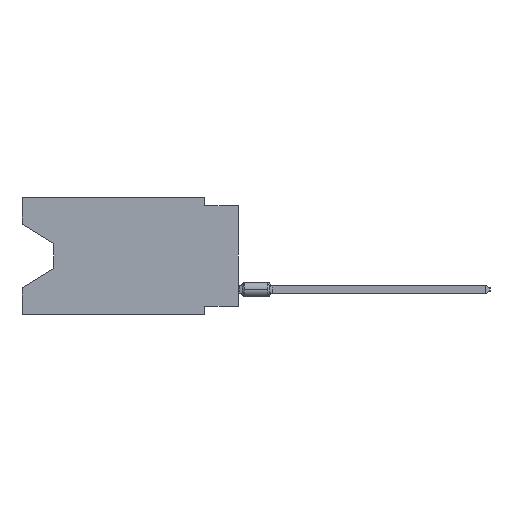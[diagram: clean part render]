
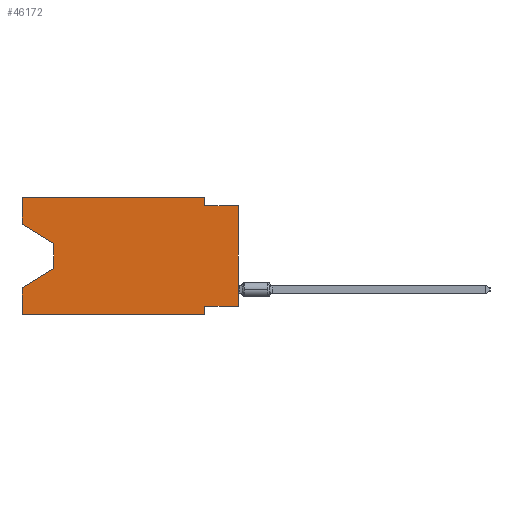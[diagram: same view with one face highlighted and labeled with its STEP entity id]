
A CAD part, left-side view. The second image highlights one B-rep face of the part: STEP entity #46172.
In plain terms, the highlighted planar face has unit normal (-1, 0, 0).
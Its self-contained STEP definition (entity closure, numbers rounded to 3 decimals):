
#573 = CARTESIAN_POINT ( 'NONE',  ( 0., 16.383, 0. ) ) ;
#797 = CARTESIAN_POINT ( 'NONE',  ( 0., 0., 0. ) ) ;
#1622 = FACE_OUTER_BOUND ( 'NONE', #34906, .T. ) ;
#1699 = ORIENTED_EDGE ( 'NONE', *, *, #53147, .F. ) ;
#1901 = ORIENTED_EDGE ( 'NONE', *, *, #46007, .F. ) ;
#3218 = VECTOR ( 'NONE', #59143, 1000. ) ;
#4753 = CARTESIAN_POINT ( 'NONE',  ( 0., 2.54, -8.89 ) ) ;
#4857 = ORIENTED_EDGE ( 'NONE', *, *, #44909, .F. ) ;
#4880 = CARTESIAN_POINT ( 'NONE',  ( 0., 2.54, -8.255 ) ) ;
#5239 = VERTEX_POINT ( 'NONE', #45162 ) ;
#5913 = DIRECTION ( 'NONE',  ( 0., 0., -1. ) ) ;
#6599 = VECTOR ( 'NONE', #42693, 1000. ) ;
#9286 = VERTEX_POINT ( 'NONE', #69932 ) ;
#9695 = LINE ( 'NONE', #57560, #27453 ) ;
#13387 = LINE ( 'NONE', #573, #32443 ) ;
#13675 = DIRECTION ( 'NONE',  ( 0., 0.855, -0.519 ) ) ;
#13773 = ORIENTED_EDGE ( 'NONE', *, *, #48867, .T. ) ;
#15728 = EDGE_CURVE ( 'NONE', #70137, #43646, #58070, .T. ) ;
#15932 = DIRECTION ( 'NONE',  ( 0., -1., 0. ) ) ;
#17198 = CARTESIAN_POINT ( 'NONE',  ( 0., 16.383, 0. ) ) ;
#17421 = CARTESIAN_POINT ( 'NONE',  ( 0., 16.383, 0. ) ) ;
#17862 = ORIENTED_EDGE ( 'NONE', *, *, #40400, .T. ) ;
#17984 = CARTESIAN_POINT ( 'NONE',  ( 0., 13.97, -5.385 ) ) ;
#18356 = DIRECTION ( 'NONE',  ( 0., 0., 1. ) ) ;
#19121 = CARTESIAN_POINT ( 'NONE',  ( 0., 16.383, 0. ) ) ;
#20349 = CARTESIAN_POINT ( 'NONE',  ( 0., 13.97, -3.505 ) ) ;
#23929 = VERTEX_POINT ( 'NONE', #45137 ) ;
#24538 = DIRECTION ( 'NONE',  ( 0., 0., 1. ) ) ;
#25149 = VERTEX_POINT ( 'NONE', #27249 ) ;
#26267 = VECTOR ( 'NONE', #41177, 1000. ) ;
#26538 = EDGE_CURVE ( 'NONE', #53308, #5239, #53725, .T. ) ;
#27249 = CARTESIAN_POINT ( 'NONE',  ( 0., 13.97, -5.385 ) ) ;
#27453 = VECTOR ( 'NONE', #15932, 1000. ) ;
#30924 = VECTOR ( 'NONE', #5913, 1000. ) ;
#32443 = VECTOR ( 'NONE', #37129, 1000. ) ;
#32713 = ORIENTED_EDGE ( 'NONE', *, *, #26538, .F. ) ;
#34519 = ORIENTED_EDGE ( 'NONE', *, *, #42650, .F. ) ;
#34906 = EDGE_LOOP ( 'NONE', ( #13773, #42897, #68142, #4857, #58822, #54046, #1901, #17862, #32713, #66331, #34519, #1699 ) ) ;
#37129 = DIRECTION ( 'NONE',  ( 0., -1., 0. ) ) ;
#40400 = EDGE_CURVE ( 'NONE', #71248, #5239, #59157, .T. ) ;
#40989 = VECTOR ( 'NONE', #24538, 1000. ) ;
#41177 = DIRECTION ( 'NONE',  ( 0., 0., 1. ) ) ;
#41263 = LINE ( 'NONE', #53324, #3218 ) ;
#42650 = EDGE_CURVE ( 'NONE', #49979, #69189, #13387, .T. ) ;
#42693 = DIRECTION ( 'NONE',  ( 0., 1., 0. ) ) ;
#42897 = ORIENTED_EDGE ( 'NONE', *, *, #61848, .T. ) ;
#42988 = EDGE_CURVE ( 'NONE', #25149, #9286, #54547, .T. ) ;
#43270 = DIRECTION ( 'NONE',  ( 0., 0., -1. ) ) ;
#43273 = CARTESIAN_POINT ( 'NONE',  ( 0., 2.54, -0.635 ) ) ;
#43646 = VERTEX_POINT ( 'NONE', #53907 ) ;
#44909 = EDGE_CURVE ( 'NONE', #23929, #9286, #70735, .T. ) ;
#45137 = CARTESIAN_POINT ( 'NONE',  ( 0., 16.383, -8.89 ) ) ;
#45162 = CARTESIAN_POINT ( 'NONE',  ( 0., 0., -0.635 ) ) ;
#45393 = DIRECTION ( 'NONE',  ( 0., 0., -1. ) ) ;
#46007 = EDGE_CURVE ( 'NONE', #71248, #70137, #71869, .T. ) ;
#46172 = ADVANCED_FACE ( 'NONE', ( #1622 ), #48698, .F. ) ;
#48264 = CARTESIAN_POINT ( 'NONE',  ( 0., 0., -0.635 ) ) ;
#48698 = PLANE ( 'NONE',  #62473 ) ;
#48867 = EDGE_CURVE ( 'NONE', #67295, #50625, #41263, .T. ) ;
#49087 = DIRECTION ( 'NONE',  ( 1., 0., 0. ) ) ;
#49979 = VERTEX_POINT ( 'NONE', #17198 ) ;
#50625 = VERTEX_POINT ( 'NONE', #20349 ) ;
#53147 = EDGE_CURVE ( 'NONE', #67295, #49979, #71288, .T. ) ;
#53308 = VERTEX_POINT ( 'NONE', #43273 ) ;
#53324 = CARTESIAN_POINT ( 'NONE',  ( 0., 16.383, -2.038 ) ) ;
#53725 = LINE ( 'NONE', #48264, #71675 ) ;
#53907 = CARTESIAN_POINT ( 'NONE',  ( 0., 2.54, -8.89 ) ) ;
#54046 = ORIENTED_EDGE ( 'NONE', *, *, #15728, .F. ) ;
#54547 = LINE ( 'NONE', #17984, #74517 ) ;
#55778 = VECTOR ( 'NONE', #18356, 1000. ) ;
#56855 = CARTESIAN_POINT ( 'NONE',  ( 0., 2.54, 0. ) ) ;
#57560 = CARTESIAN_POINT ( 'NONE',  ( 0., 16.383, -8.89 ) ) ;
#58070 = LINE ( 'NONE', #4753, #30924 ) ;
#58822 = ORIENTED_EDGE ( 'NONE', *, *, #74525, .T. ) ;
#58921 = CARTESIAN_POINT ( 'NONE',  ( 0., 16.383, -2.038 ) ) ;
#59143 = DIRECTION ( 'NONE',  ( 0., -0.855, -0.519 ) ) ;
#59157 = LINE ( 'NONE', #797, #40989 ) ;
#59520 = EDGE_CURVE ( 'NONE', #69189, #53308, #70966, .T. ) ;
#59994 = CARTESIAN_POINT ( 'NONE',  ( 0., 16.383, 0. ) ) ;
#61735 = VECTOR ( 'NONE', #45393, 1000. ) ;
#61848 = EDGE_CURVE ( 'NONE', #50625, #25149, #69508, .T. ) ;
#62473 = AXIS2_PLACEMENT_3D ( 'NONE', #19121, #49087, #43270 ) ;
#64355 = DIRECTION ( 'NONE',  ( 0., 0., -1. ) ) ;
#64430 = CARTESIAN_POINT ( 'NONE',  ( 0., 13.97, -3.505 ) ) ;
#65195 = VECTOR ( 'NONE', #64355, 1000. ) ;
#66331 = ORIENTED_EDGE ( 'NONE', *, *, #59520, .F. ) ;
#67295 = VERTEX_POINT ( 'NONE', #58921 ) ;
#68142 = ORIENTED_EDGE ( 'NONE', *, *, #42988, .T. ) ;
#69189 = VERTEX_POINT ( 'NONE', #56855 ) ;
#69508 = LINE ( 'NONE', #64430, #61735 ) ;
#69932 = CARTESIAN_POINT ( 'NONE',  ( 0., 16.383, -6.852 ) ) ;
#69965 = CARTESIAN_POINT ( 'NONE',  ( 0., 0., -8.255 ) ) ;
#70137 = VERTEX_POINT ( 'NONE', #4880 ) ;
#70735 = LINE ( 'NONE', #17421, #26267 ) ;
#70966 = LINE ( 'NONE', #76027, #65195 ) ;
#71248 = VERTEX_POINT ( 'NONE', #69965 ) ;
#71288 = LINE ( 'NONE', #59994, #55778 ) ;
#71675 = VECTOR ( 'NONE', #71991, 1000. ) ;
#71869 = LINE ( 'NONE', #73416, #6599 ) ;
#71991 = DIRECTION ( 'NONE',  ( 0., -1., 0. ) ) ;
#73416 = CARTESIAN_POINT ( 'NONE',  ( 0., 0., -8.255 ) ) ;
#74517 = VECTOR ( 'NONE', #13675, 1000. ) ;
#74525 = EDGE_CURVE ( 'NONE', #23929, #43646, #9695, .T. ) ;
#76027 = CARTESIAN_POINT ( 'NONE',  ( 0., 2.54, 0. ) ) ;
